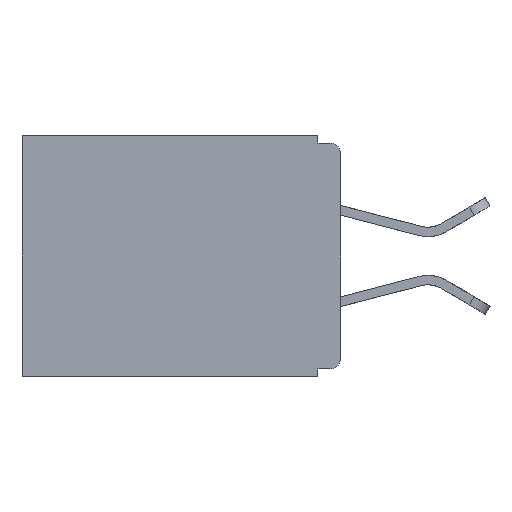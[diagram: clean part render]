
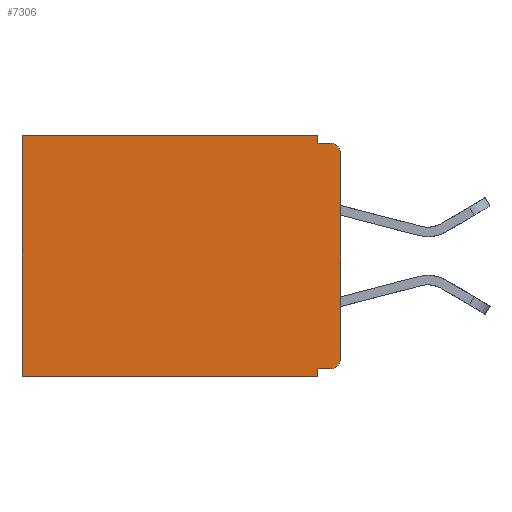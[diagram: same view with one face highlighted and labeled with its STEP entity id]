
A CAD part, left-side view. The second image highlights one B-rep face of the part: STEP entity #7306.
In plain terms, the highlighted planar face has unit normal (-1, 0, 0).
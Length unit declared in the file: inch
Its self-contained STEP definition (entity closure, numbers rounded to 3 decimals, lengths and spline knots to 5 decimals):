
#869 = CARTESIAN_POINT ( 'NONE',  ( 0.3, 0.437, 0. ) ) ;
#913 = DIRECTION ( 'NONE',  ( -1., 0., 0. ) ) ;
#1535 = CARTESIAN_POINT ( 'NONE',  ( 0.3, 0., -0.33 ) ) ;
#2115 = VERTEX_POINT ( 'NONE', #32598 ) ;
#2484 = VERTEX_POINT ( 'NONE', #4182 ) ;
#2607 = CARTESIAN_POINT ( 'NONE',  ( 0.3, 0., -0.33 ) ) ;
#2656 = ORIENTED_EDGE ( 'NONE', *, *, #17564, .F. ) ;
#2918 = VERTEX_POINT ( 'NONE', #869 ) ;
#3467 = CARTESIAN_POINT ( 'NONE',  ( 0.3, 0.015, -0.01 ) ) ;
#3709 = DIRECTION ( 'NONE',  ( 0., 0., -1. ) ) ;
#3969 = DIRECTION ( 'NONE',  ( 0., -1., 0. ) ) ;
#4182 = CARTESIAN_POINT ( 'NONE',  ( 0.3, 0.031, 0. ) ) ;
#4308 = DIRECTION ( 'NONE',  ( 0., 0., -1. ) ) ;
#4381 = EDGE_LOOP ( 'NONE', ( #12186, #18611, #10101, #2656, #8329, #28086, #4803, #18646, #23146, #16087 ) ) ;
#4515 = VECTOR ( 'NONE', #13414, 39.37008 ) ;
#4803 = ORIENTED_EDGE ( 'NONE', *, *, #27273, .F. ) ;
#5524 = VERTEX_POINT ( 'NONE', #10024 ) ;
#5625 = LINE ( 'NONE', #1535, #19439 ) ;
#6357 = CARTESIAN_POINT ( 'NONE',  ( 0.3, 0.031, -0.01 ) ) ;
#7306 = ADVANCED_FACE ( 'NONE', ( #15239 ), #15379, .F. ) ;
#8190 = DIRECTION ( 'NONE',  ( -1., 0., 0. ) ) ;
#8329 = ORIENTED_EDGE ( 'NONE', *, *, #24045, .T. ) ;
#8338 = CARTESIAN_POINT ( 'NONE',  ( 0.3, 0.031, -0.33 ) ) ;
#8872 = AXIS2_PLACEMENT_3D ( 'NONE', #24346, #8190, #27023 ) ;
#9410 = VERTEX_POINT ( 'NONE', #6357 ) ;
#9551 = CARTESIAN_POINT ( 'NONE',  ( 0.3, 0.437, -0.33 ) ) ;
#9608 = CARTESIAN_POINT ( 'NONE',  ( 0.3, 0., -0.01 ) ) ;
#9873 = AXIS2_PLACEMENT_3D ( 'NONE', #17522, #913, #20187 ) ;
#10024 = CARTESIAN_POINT ( 'NONE',  ( 0.3, 0., -0.305 ) ) ;
#10101 = ORIENTED_EDGE ( 'NONE', *, *, #21762, .F. ) ;
#10549 = DIRECTION ( 'NONE',  ( 0., 1., 0. ) ) ;
#10656 = VERTEX_POINT ( 'NONE', #19765 ) ;
#11072 = EDGE_CURVE ( 'NONE', #2115, #26346, #32317, .T. ) ;
#11990 = CARTESIAN_POINT ( 'NONE',  ( 0.3, 0.031, 0. ) ) ;
#12027 = CARTESIAN_POINT ( 'NONE',  ( 0.3, 0.031, -0.32 ) ) ;
#12186 = ORIENTED_EDGE ( 'NONE', *, *, #29599, .F. ) ;
#12221 = VERTEX_POINT ( 'NONE', #9551 ) ;
#13414 = DIRECTION ( 'NONE',  ( 0., 1., 0. ) ) ;
#14191 = VERTEX_POINT ( 'NONE', #33884 ) ;
#14405 = DIRECTION ( 'NONE',  ( 0., 0., -1. ) ) ;
#14589 = DIRECTION ( 'NONE',  ( 1., 0., 0. ) ) ;
#15076 = CARTESIAN_POINT ( 'NONE',  ( 0.3, 0., -0.33 ) ) ;
#15239 = FACE_OUTER_BOUND ( 'NONE', #4381, .T. ) ;
#15379 = PLANE ( 'NONE',  #21226 ) ;
#16087 = ORIENTED_EDGE ( 'NONE', *, *, #19481, .T. ) ;
#16385 = VECTOR ( 'NONE', #3969, 39.37008 ) ;
#16703 = EDGE_CURVE ( 'NONE', #2918, #12221, #30934, .T. ) ;
#17051 = CIRCLE ( 'NONE', #8872, 0.015 ) ;
#17522 = CARTESIAN_POINT ( 'NONE',  ( 0.3, 0.015, -0.305 ) ) ;
#17564 = EDGE_CURVE ( 'NONE', #2484, #9410, #19394, .T. ) ;
#18611 = ORIENTED_EDGE ( 'NONE', *, *, #33340, .T. ) ;
#18646 = ORIENTED_EDGE ( 'NONE', *, *, #24145, .F. ) ;
#19181 = LINE ( 'NONE', #24062, #26143 ) ;
#19394 = LINE ( 'NONE', #11990, #31705 ) ;
#19439 = VECTOR ( 'NONE', #4308, 39.37008 ) ;
#19481 = EDGE_CURVE ( 'NONE', #2115, #5524, #26639, .T. ) ;
#19765 = CARTESIAN_POINT ( 'NONE',  ( 0.3, 0., -0.025 ) ) ;
#19776 = VECTOR ( 'NONE', #24377, 39.37008 ) ;
#20187 = DIRECTION ( 'NONE',  ( 0., 0., -1. ) ) ;
#21226 = AXIS2_PLACEMENT_3D ( 'NONE', #15076, #14589, #14405 ) ;
#21762 = EDGE_CURVE ( 'NONE', #9410, #26945, #22833, .T. ) ;
#22833 = LINE ( 'NONE', #9608, #16385 ) ;
#23146 = ORIENTED_EDGE ( 'NONE', *, *, #11072, .F. ) ;
#23657 = VECTOR ( 'NONE', #27165, 39.37008 ) ;
#23666 = CARTESIAN_POINT ( 'NONE',  ( 0.3, 0.437, -0.33 ) ) ;
#24045 = EDGE_CURVE ( 'NONE', #2484, #2918, #19181, .T. ) ;
#24062 = CARTESIAN_POINT ( 'NONE',  ( 0.3, 0., 0. ) ) ;
#24145 = EDGE_CURVE ( 'NONE', #26346, #14191, #29027, .T. ) ;
#24346 = CARTESIAN_POINT ( 'NONE',  ( 0.3, 0.015, -0.025 ) ) ;
#24377 = DIRECTION ( 'NONE',  ( 0., 1., 0. ) ) ;
#26143 = VECTOR ( 'NONE', #10549, 39.37008 ) ;
#26346 = VERTEX_POINT ( 'NONE', #12027 ) ;
#26639 = CIRCLE ( 'NONE', #9873, 0.015 ) ;
#26945 = VERTEX_POINT ( 'NONE', #3467 ) ;
#27023 = DIRECTION ( 'NONE',  ( 0., 0., -1. ) ) ;
#27165 = DIRECTION ( 'NONE',  ( 0., 0., -1. ) ) ;
#27273 = EDGE_CURVE ( 'NONE', #14191, #12221, #32890, .T. ) ;
#28086 = ORIENTED_EDGE ( 'NONE', *, *, #16703, .T. ) ;
#29027 = LINE ( 'NONE', #8338, #23657 ) ;
#29599 = EDGE_CURVE ( 'NONE', #10656, #5524, #5625, .T. ) ;
#30106 = VECTOR ( 'NONE', #34098, 39.37008 ) ;
#30934 = LINE ( 'NONE', #23666, #30106 ) ;
#31705 = VECTOR ( 'NONE', #3709, 39.37008 ) ;
#31999 = CARTESIAN_POINT ( 'NONE',  ( 0.3, 0., -0.32 ) ) ;
#32317 = LINE ( 'NONE', #31999, #4515 ) ;
#32598 = CARTESIAN_POINT ( 'NONE',  ( 0.3, 0.015, -0.32 ) ) ;
#32890 = LINE ( 'NONE', #2607, #19776 ) ;
#33340 = EDGE_CURVE ( 'NONE', #10656, #26945, #17051, .T. ) ;
#33884 = CARTESIAN_POINT ( 'NONE',  ( 0.3, 0.031, -0.33 ) ) ;
#34098 = DIRECTION ( 'NONE',  ( 0., 0., -1. ) ) ;
